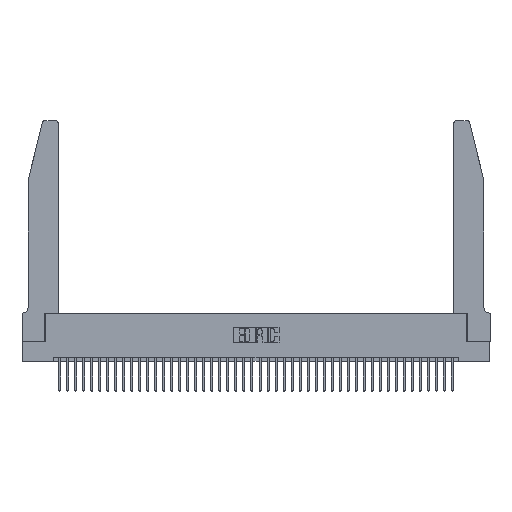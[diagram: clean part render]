
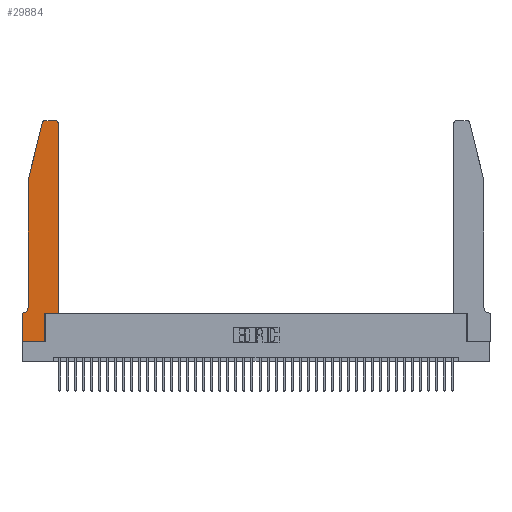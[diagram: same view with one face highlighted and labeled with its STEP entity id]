
A CAD part, top view. The second image highlights one B-rep face of the part: STEP entity #29884.
In plain terms, the highlighted planar face has unit normal (0, 0, 1).
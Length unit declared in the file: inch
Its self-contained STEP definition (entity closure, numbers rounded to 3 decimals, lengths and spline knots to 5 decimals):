
#202 = CIRCLE ( 'NONE', #32036, 0.07 ) ;
#627 = CARTESIAN_POINT ( 'NONE',  ( 0., 0., 0.37 ) ) ;
#907 = EDGE_CURVE ( 'NONE', #37951, #23051, #33625, .T. ) ;
#1672 = LINE ( 'NONE', #17523, #23459 ) ;
#1692 = CARTESIAN_POINT ( 'NONE',  ( 0.284, 2.75, 0.37 ) ) ;
#1976 = CARTESIAN_POINT ( 'NONE',  ( 0.0055, 0.42, 0.37 ) ) ;
#3427 = CARTESIAN_POINT ( 'NONE',  ( 0.25487, 2.72718, 0.37 ) ) ;
#3851 = DIRECTION ( 'NONE',  ( 1., 0., 0. ) ) ;
#4904 = VECTOR ( 'NONE', #29803, 39.37008 ) ;
#5427 = DIRECTION ( 'NONE',  ( -1., 0., 0. ) ) ;
#5490 = ORIENTED_EDGE ( 'NONE', *, *, #19796, .T. ) ;
#6611 = VECTOR ( 'NONE', #3851, 39.37008 ) ;
#7371 = LINE ( 'NONE', #30092, #34957 ) ;
#7649 = DIRECTION ( 'NONE',  ( 0., 0., 1. ) ) ;
#7722 = CARTESIAN_POINT ( 'NONE',  ( 0., 0., 0.37 ) ) ;
#8015 = ORIENTED_EDGE ( 'NONE', *, *, #34002, .T. ) ;
#8286 = CARTESIAN_POINT ( 'NONE',  ( 0.4205, 2.75, 0.37 ) ) ;
#8315 = ORIENTED_EDGE ( 'NONE', *, *, #10424, .T. ) ;
#9205 = EDGE_CURVE ( 'NONE', #18937, #30442, #33467, .T. ) ;
#9773 = ORIENTED_EDGE ( 'NONE', *, *, #42208, .T. ) ;
#9819 = ORIENTED_EDGE ( 'NONE', *, *, #28544, .T. ) ;
#10267 = VECTOR ( 'NONE', #25836, 39.37008 ) ;
#10424 = EDGE_CURVE ( 'NONE', #19262, #27774, #1672, .T. ) ;
#10554 = DIRECTION ( 'NONE',  ( 0., 0., 1. ) ) ;
#10696 = DIRECTION ( 'NONE',  ( -1., 0., 0. ) ) ;
#11952 = DIRECTION ( 'NONE',  ( 0., 1., 0. ) ) ;
#12245 = DIRECTION ( 'NONE',  ( 0., 1., 0. ) ) ;
#13217 = CARTESIAN_POINT ( 'NONE',  ( 0., 0., 0.37 ) ) ;
#13277 = VECTOR ( 'NONE', #23889, 39.37008 ) ;
#13287 = ORIENTED_EDGE ( 'NONE', *, *, #28857, .T. ) ;
#14089 = LINE ( 'NONE', #13217, #31794 ) ;
#14212 = VERTEX_POINT ( 'NONE', #7722 ) ;
#15071 = LINE ( 'NONE', #31312, #30675 ) ;
#15896 = DIRECTION ( 'NONE',  ( 0., 0., 1. ) ) ;
#17523 = CARTESIAN_POINT ( 'NONE',  ( 0.2605, 2.75, 0.37 ) ) ;
#17736 = CARTESIAN_POINT ( 'NONE',  ( 0., 0.35, 0.37 ) ) ;
#18937 = VERTEX_POINT ( 'NONE', #41390 ) ;
#19026 = CARTESIAN_POINT ( 'NONE',  ( 0.4505, 2.72, 0.37 ) ) ;
#19262 = VERTEX_POINT ( 'NONE', #8286 ) ;
#19796 = EDGE_CURVE ( 'NONE', #29214, #19262, #32868, .T. ) ;
#20353 = FACE_OUTER_BOUND ( 'NONE', #30962, .T. ) ;
#21612 = AXIS2_PLACEMENT_3D ( 'NONE', #23083, #10554, #37249 ) ;
#22505 = CARTESIAN_POINT ( 'NONE',  ( 0.4505, 0.35, 0.37 ) ) ;
#23051 = VERTEX_POINT ( 'NONE', #37735 ) ;
#23083 = CARTESIAN_POINT ( 'NONE',  ( 0.284, 2.72, 0.37 ) ) ;
#23277 = VERTEX_POINT ( 'NONE', #22505 ) ;
#23459 = VECTOR ( 'NONE', #10696, 39.37008 ) ;
#23645 = VERTEX_POINT ( 'NONE', #28597 ) ;
#23889 = DIRECTION ( 'NONE',  ( 1., 0., 0. ) ) ;
#24687 = EDGE_CURVE ( 'NONE', #14212, #23645, #28421, .T. ) ;
#24904 = AXIS2_PLACEMENT_3D ( 'NONE', #32472, #15896, #42623 ) ;
#24987 = CIRCLE ( 'NONE', #21612, 0.03 ) ;
#25592 = VECTOR ( 'NONE', #12245, 39.37008 ) ;
#25701 = CARTESIAN_POINT ( 'NONE',  ( 0.0755, 2., 0.37 ) ) ;
#25836 = DIRECTION ( 'NONE',  ( 0., -1., 0. ) ) ;
#25978 = DIRECTION ( 'NONE',  ( 0., -1., 0. ) ) ;
#27523 = PLANE ( 'NONE',  #36778 ) ;
#27774 = VERTEX_POINT ( 'NONE', #1692 ) ;
#28421 = LINE ( 'NONE', #627, #6611 ) ;
#28544 = EDGE_CURVE ( 'NONE', #23277, #29214, #34441, .T. ) ;
#28597 = CARTESIAN_POINT ( 'NONE',  ( 0.2865, 0., 0.37 ) ) ;
#28774 = ORIENTED_EDGE ( 'NONE', *, *, #29492, .T. ) ;
#28857 = EDGE_CURVE ( 'NONE', #30791, #37951, #7371, .T. ) ;
#29214 = VERTEX_POINT ( 'NONE', #19026 ) ;
#29492 = EDGE_CURVE ( 'NONE', #30442, #14212, #14089, .T. ) ;
#29803 = DIRECTION ( 'NONE',  ( -1., 0., 0. ) ) ;
#29884 = ADVANCED_FACE ( 'NONE', ( #20353 ), #27523, .T. ) ;
#30092 = CARTESIAN_POINT ( 'NONE',  ( 0.0755, 2., 0.37 ) ) ;
#30323 = CARTESIAN_POINT ( 'NONE',  ( 0.4505, 0.35, 0.37 ) ) ;
#30442 = VERTEX_POINT ( 'NONE', #17736 ) ;
#30675 = VECTOR ( 'NONE', #11952, 39.37008 ) ;
#30750 = DIRECTION ( 'NONE',  ( 1., 0., 0. ) ) ;
#30791 = VERTEX_POINT ( 'NONE', #3427 ) ;
#30962 = EDGE_LOOP ( 'NONE', ( #8315, #8015, #13287, #32169, #34214, #33883, #28774, #42007, #9773, #42841, #9819, #5490 ) ) ;
#31312 = CARTESIAN_POINT ( 'NONE',  ( 0.2865, 0.35, 0.37 ) ) ;
#31794 = VECTOR ( 'NONE', #25978, 39.37008 ) ;
#32036 = AXIS2_PLACEMENT_3D ( 'NONE', #1976, #38785, #5427 ) ;
#32169 = ORIENTED_EDGE ( 'NONE', *, *, #907, .T. ) ;
#32472 = CARTESIAN_POINT ( 'NONE',  ( 0.4205, 2.72, 0.37 ) ) ;
#32516 = CARTESIAN_POINT ( 'NONE',  ( 0.0755, 2., 0.37 ) ) ;
#32868 = CIRCLE ( 'NONE', #24904, 0.03 ) ;
#33467 = LINE ( 'NONE', #36286, #4904 ) ;
#33610 = VERTEX_POINT ( 'NONE', #40494 ) ;
#33625 = LINE ( 'NONE', #25701, #10267 ) ;
#33824 = DIRECTION ( 'NONE',  ( -0.239, -0.971, 0. ) ) ;
#33883 = ORIENTED_EDGE ( 'NONE', *, *, #9205, .T. ) ;
#34002 = EDGE_CURVE ( 'NONE', #27774, #30791, #24987, .T. ) ;
#34214 = ORIENTED_EDGE ( 'NONE', *, *, #37078, .T. ) ;
#34441 = LINE ( 'NONE', #35215, #25592 ) ;
#34529 = CARTESIAN_POINT ( 'NONE',  ( 0., 0.35, 0.37 ) ) ;
#34957 = VECTOR ( 'NONE', #33824, 39.37008 ) ;
#35215 = CARTESIAN_POINT ( 'NONE',  ( 0.4505, 0.35, 0.37 ) ) ;
#36103 = EDGE_CURVE ( 'NONE', #33610, #23277, #36635, .T. ) ;
#36286 = CARTESIAN_POINT ( 'NONE',  ( 0.0755, 0.35, 0.37 ) ) ;
#36635 = LINE ( 'NONE', #30323, #13277 ) ;
#36778 = AXIS2_PLACEMENT_3D ( 'NONE', #34529, #7649, #30750 ) ;
#37078 = EDGE_CURVE ( 'NONE', #23051, #18937, #202, .T. ) ;
#37249 = DIRECTION ( 'NONE',  ( 1., 0., 0. ) ) ;
#37735 = CARTESIAN_POINT ( 'NONE',  ( 0.0755, 0.42, 0.37 ) ) ;
#37951 = VERTEX_POINT ( 'NONE', #32516 ) ;
#38785 = DIRECTION ( 'NONE',  ( 0., 0., -1. ) ) ;
#40494 = CARTESIAN_POINT ( 'NONE',  ( 0.2865, 0.35, 0.37 ) ) ;
#41390 = CARTESIAN_POINT ( 'NONE',  ( 0.0055, 0.35, 0.37 ) ) ;
#42007 = ORIENTED_EDGE ( 'NONE', *, *, #24687, .T. ) ;
#42208 = EDGE_CURVE ( 'NONE', #23645, #33610, #15071, .T. ) ;
#42623 = DIRECTION ( 'NONE',  ( 1., 0., 0. ) ) ;
#42841 = ORIENTED_EDGE ( 'NONE', *, *, #36103, .T. ) ;
